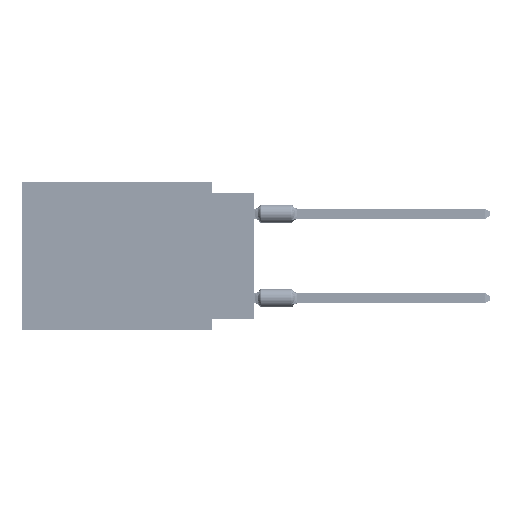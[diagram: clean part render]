
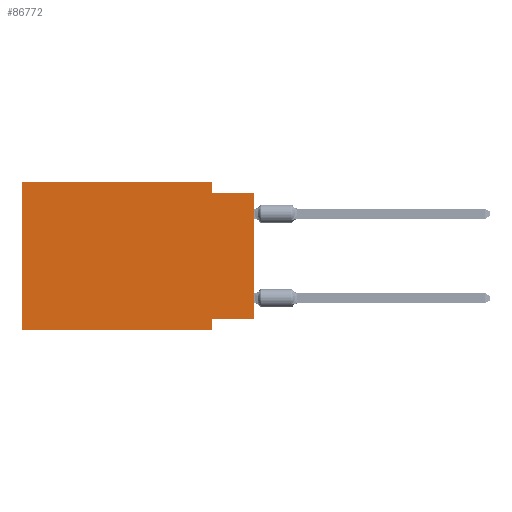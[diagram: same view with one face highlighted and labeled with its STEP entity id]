
A CAD part, left-side view. The second image highlights one B-rep face of the part: STEP entity #86772.
In plain terms, the highlighted planar face has unit normal (-1, 0, 0).
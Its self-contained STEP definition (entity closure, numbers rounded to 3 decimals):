
#2040 = CARTESIAN_POINT ( 'NONE',  ( 0., 13.97, 0. ) ) ;
#5144 = DIRECTION ( 'NONE',  ( 0., -1., 0. ) ) ;
#6719 = VERTEX_POINT ( 'NONE', #28993 ) ;
#7011 = ORIENTED_EDGE ( 'NONE', *, *, #66573, .F. ) ;
#9649 = DIRECTION ( 'NONE',  ( 0., 0., -1. ) ) ;
#9860 = ORIENTED_EDGE ( 'NONE', *, *, #33480, .F. ) ;
#10230 = CARTESIAN_POINT ( 'NONE',  ( 0., 13.97, 0. ) ) ;
#10576 = CARTESIAN_POINT ( 'NONE',  ( 0., 2.54, 0. ) ) ;
#11274 = EDGE_CURVE ( 'NONE', #34766, #14353, #31451, .T. ) ;
#12036 = CARTESIAN_POINT ( 'NONE',  ( 0., 0., -8.255 ) ) ;
#12616 = VECTOR ( 'NONE', #22460, 1000. ) ;
#14353 = VERTEX_POINT ( 'NONE', #90049 ) ;
#15175 = VERTEX_POINT ( 'NONE', #21017 ) ;
#15234 = CARTESIAN_POINT ( 'NONE',  ( 0., 2.54, -0.635 ) ) ;
#15347 = DIRECTION ( 'NONE',  ( 0., 0., -1. ) ) ;
#16531 = AXIS2_PLACEMENT_3D ( 'NONE', #2040, #31472, #15347 ) ;
#16935 = EDGE_LOOP ( 'NONE', ( #57277, #18230, #9860, #23504, #59941, #28885, #31996, #7011 ) ) ;
#17999 = VERTEX_POINT ( 'NONE', #55651 ) ;
#18230 = ORIENTED_EDGE ( 'NONE', *, *, #56851, .F. ) ;
#19340 = DIRECTION ( 'NONE',  ( 0., 0., 1. ) ) ;
#19717 = VECTOR ( 'NONE', #55688, 1000. ) ;
#21017 = CARTESIAN_POINT ( 'NONE',  ( 0., 2.54, -8.89 ) ) ;
#22460 = DIRECTION ( 'NONE',  ( 0., -1., 0. ) ) ;
#22516 = EDGE_CURVE ( 'NONE', #6719, #34766, #28390, .T. ) ;
#22946 = LINE ( 'NONE', #10576, #47919 ) ;
#23504 = ORIENTED_EDGE ( 'NONE', *, *, #11274, .F. ) ;
#25969 = VECTOR ( 'NONE', #82359, 1000. ) ;
#28390 = LINE ( 'NONE', #63568, #73950 ) ;
#28885 = ORIENTED_EDGE ( 'NONE', *, *, #71396, .T. ) ;
#28993 = CARTESIAN_POINT ( 'NONE',  ( 0., 13.97, -8.89 ) ) ;
#31326 = VERTEX_POINT ( 'NONE', #82309 ) ;
#31451 = LINE ( 'NONE', #60433, #12616 ) ;
#31472 = DIRECTION ( 'NONE',  ( 1., 0., 0. ) ) ;
#31996 = ORIENTED_EDGE ( 'NONE', *, *, #88044, .F. ) ;
#32568 = VECTOR ( 'NONE', #83193, 1000. ) ;
#33480 = EDGE_CURVE ( 'NONE', #14353, #52351, #22946, .T. ) ;
#34766 = VERTEX_POINT ( 'NONE', #10230 ) ;
#40242 = LINE ( 'NONE', #84413, #56170 ) ;
#41239 = LINE ( 'NONE', #70203, #83921 ) ;
#42247 = EDGE_CURVE ( 'NONE', #17999, #66168, #40242, .T. ) ;
#42635 = DIRECTION ( 'NONE',  ( 0., 0., 1. ) ) ;
#45272 = LINE ( 'NONE', #83247, #19717 ) ;
#47919 = VECTOR ( 'NONE', #9649, 1000. ) ;
#48123 = LINE ( 'NONE', #12036, #25969 ) ;
#48234 = CARTESIAN_POINT ( 'NONE',  ( 0., 0., -0.635 ) ) ;
#52351 = VERTEX_POINT ( 'NONE', #15234 ) ;
#55651 = CARTESIAN_POINT ( 'NONE',  ( 0., 0., -8.255 ) ) ;
#55688 = DIRECTION ( 'NONE',  ( 0., 0., -1. ) ) ;
#56170 = VECTOR ( 'NONE', #19340, 1000. ) ;
#56851 = EDGE_CURVE ( 'NONE', #52351, #66168, #41239, .T. ) ;
#57277 = ORIENTED_EDGE ( 'NONE', *, *, #42247, .T. ) ;
#59941 = ORIENTED_EDGE ( 'NONE', *, *, #22516, .F. ) ;
#59992 = PLANE ( 'NONE',  #16531 ) ;
#60433 = CARTESIAN_POINT ( 'NONE',  ( 0., 13.97, 0. ) ) ;
#61831 = CARTESIAN_POINT ( 'NONE',  ( 0., 13.97, -8.89 ) ) ;
#63568 = CARTESIAN_POINT ( 'NONE',  ( 0., 13.97, 0. ) ) ;
#66168 = VERTEX_POINT ( 'NONE', #48234 ) ;
#66573 = EDGE_CURVE ( 'NONE', #17999, #31326, #48123, .T. ) ;
#67066 = LINE ( 'NONE', #61831, #32568 ) ;
#67105 = FACE_OUTER_BOUND ( 'NONE', #16935, .T. ) ;
#70203 = CARTESIAN_POINT ( 'NONE',  ( 0., 0., -0.635 ) ) ;
#71396 = EDGE_CURVE ( 'NONE', #6719, #15175, #67066, .T. ) ;
#73950 = VECTOR ( 'NONE', #42635, 1000. ) ;
#82309 = CARTESIAN_POINT ( 'NONE',  ( 0., 2.54, -8.255 ) ) ;
#82359 = DIRECTION ( 'NONE',  ( 0., 1., 0. ) ) ;
#83193 = DIRECTION ( 'NONE',  ( 0., -1., 0. ) ) ;
#83247 = CARTESIAN_POINT ( 'NONE',  ( 0., 2.54, -8.89 ) ) ;
#83921 = VECTOR ( 'NONE', #5144, 1000. ) ;
#84413 = CARTESIAN_POINT ( 'NONE',  ( 0., 0., 0. ) ) ;
#86772 = ADVANCED_FACE ( 'NONE', ( #67105 ), #59992, .F. ) ;
#88044 = EDGE_CURVE ( 'NONE', #31326, #15175, #45272, .T. ) ;
#90049 = CARTESIAN_POINT ( 'NONE',  ( 0., 2.54, 0. ) ) ;
